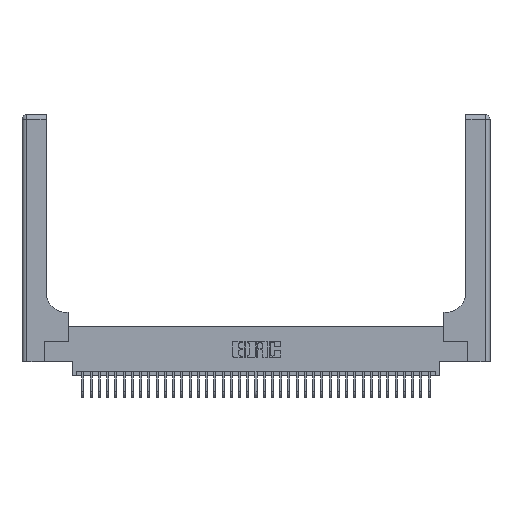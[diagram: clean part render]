
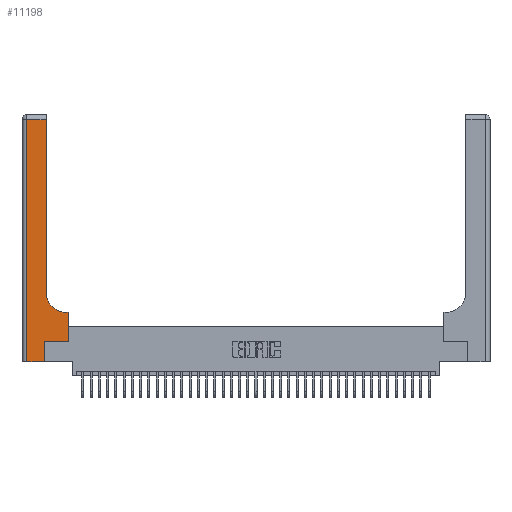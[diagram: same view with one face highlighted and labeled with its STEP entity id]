
A CAD part, top view. The second image highlights one B-rep face of the part: STEP entity #11198.
In plain terms, the highlighted planar face has unit normal (0, 0, 1).
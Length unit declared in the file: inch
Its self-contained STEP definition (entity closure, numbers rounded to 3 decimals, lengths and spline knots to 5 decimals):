
#14 = ORIENTED_EDGE ( 'NONE', *, *, #10716, .T. ) ;
#34 = VERTEX_POINT ( 'NONE', #37044 ) ;
#364 = EDGE_CURVE ( 'NONE', #31958, #33200, #26674, .T. ) ;
#442 = ORIENTED_EDGE ( 'NONE', *, *, #27554, .T. ) ;
#718 = VERTEX_POINT ( 'NONE', #11333 ) ;
#1422 = DIRECTION ( 'NONE',  ( -1., 0., 0. ) ) ;
#2027 = CARTESIAN_POINT ( 'NONE',  ( 0.5585, 0.6, 0.37 ) ) ;
#3683 = CARTESIAN_POINT ( 'NONE',  ( 0.5585, 0.25, 0.37 ) ) ;
#3736 = VERTEX_POINT ( 'NONE', #9401 ) ;
#4143 = CARTESIAN_POINT ( 'NONE',  ( 0.269, 0., 0.37 ) ) ;
#4271 = EDGE_CURVE ( 'NONE', #8091, #22768, #10926, .T. ) ;
#4682 = VERTEX_POINT ( 'NONE', #13950 ) ;
#6877 = CARTESIAN_POINT ( 'NONE',  ( 0.2915, 2.94, 0.37 ) ) ;
#7111 = DIRECTION ( 'NONE',  ( 0., 1., 0. ) ) ;
#7284 = EDGE_CURVE ( 'NONE', #4682, #8091, #32147, .T. ) ;
#7836 = VECTOR ( 'NONE', #7851, 39.37008 ) ;
#7851 = DIRECTION ( 'NONE',  ( -1., 0., 0. ) ) ;
#8091 = VERTEX_POINT ( 'NONE', #27769 ) ;
#8208 = CARTESIAN_POINT ( 'NONE',  ( 0.06, 3., 0.37 ) ) ;
#8946 = VECTOR ( 'NONE', #35458, 39.37008 ) ;
#8972 = EDGE_CURVE ( 'NONE', #34, #31958, #35555, .T. ) ;
#9401 = CARTESIAN_POINT ( 'NONE',  ( 0.2915, 0.85, 0.37 ) ) ;
#9494 = CARTESIAN_POINT ( 'NONE',  ( 0., 3., 0.37 ) ) ;
#9669 = DIRECTION ( 'NONE',  ( 1., 0., 0. ) ) ;
#9831 = CARTESIAN_POINT ( 'NONE',  ( 0.06, 0., 0.37 ) ) ;
#9869 = EDGE_CURVE ( 'NONE', #3736, #34813, #35478, .T. ) ;
#10716 = EDGE_CURVE ( 'NONE', #718, #3736, #24667, .T. ) ;
#10926 = LINE ( 'NONE', #3683, #24614 ) ;
#11183 = VECTOR ( 'NONE', #9669, 39.37008 ) ;
#11198 = ADVANCED_FACE ( 'NONE', ( #19751 ), #24074, .F. ) ;
#11333 = CARTESIAN_POINT ( 'NONE',  ( 0.5415, 0.6, 0.37 ) ) ;
#12494 = VECTOR ( 'NONE', #37082, 39.37008 ) ;
#12737 = VECTOR ( 'NONE', #1422, 39.37008 ) ;
#13571 = VECTOR ( 'NONE', #7111, 39.37008 ) ;
#13950 = CARTESIAN_POINT ( 'NONE',  ( 0.269, 0.25, 0.37 ) ) ;
#15389 = DIRECTION ( 'NONE',  ( -1., 0., 0. ) ) ;
#16310 = DIRECTION ( 'NONE',  ( 0., 0., -1. ) ) ;
#16577 = CARTESIAN_POINT ( 'NONE',  ( 0.2915, 3., 0.37 ) ) ;
#18393 = ORIENTED_EDGE ( 'NONE', *, *, #9869, .T. ) ;
#18813 = EDGE_CURVE ( 'NONE', #33200, #4682, #36606, .T. ) ;
#19751 = FACE_OUTER_BOUND ( 'NONE', #28714, .T. ) ;
#20494 = LINE ( 'NONE', #24713, #12737 ) ;
#21259 = DIRECTION ( 'NONE',  ( 0., 1., 0. ) ) ;
#22236 = AXIS2_PLACEMENT_3D ( 'NONE', #33645, #16310, #36498 ) ;
#22768 = VERTEX_POINT ( 'NONE', #2027 ) ;
#23400 = LINE ( 'NONE', #36853, #7836 ) ;
#23905 = EDGE_CURVE ( 'NONE', #34813, #34, #20494, .T. ) ;
#24074 = PLANE ( 'NONE',  #27341 ) ;
#24614 = VECTOR ( 'NONE', #21259, 39.37008 ) ;
#24667 = CIRCLE ( 'NONE', #22236, 0.25 ) ;
#24713 = CARTESIAN_POINT ( 'NONE',  ( 0., 2.94, 0.37 ) ) ;
#26674 = LINE ( 'NONE', #35755, #11183 ) ;
#26991 = VECTOR ( 'NONE', #33904, 39.37008 ) ;
#27341 = AXIS2_PLACEMENT_3D ( 'NONE', #9494, #32747, #15389 ) ;
#27554 = EDGE_CURVE ( 'NONE', #22768, #718, #23400, .T. ) ;
#27769 = CARTESIAN_POINT ( 'NONE',  ( 0.5585, 0.25, 0.37 ) ) ;
#28097 = ORIENTED_EDGE ( 'NONE', *, *, #18813, .T. ) ;
#28215 = ORIENTED_EDGE ( 'NONE', *, *, #4271, .T. ) ;
#28714 = EDGE_LOOP ( 'NONE', ( #18393, #33807, #33388, #35778, #28097, #28744, #28215, #442, #14 ) ) ;
#28744 = ORIENTED_EDGE ( 'NONE', *, *, #7284, .T. ) ;
#31313 = CARTESIAN_POINT ( 'NONE',  ( 0.269, 0., 0.37 ) ) ;
#31958 = VERTEX_POINT ( 'NONE', #9831 ) ;
#32147 = LINE ( 'NONE', #32619, #8946 ) ;
#32619 = CARTESIAN_POINT ( 'NONE',  ( 0.269, 0.25, 0.37 ) ) ;
#32747 = DIRECTION ( 'NONE',  ( 0., 0., -1. ) ) ;
#33200 = VERTEX_POINT ( 'NONE', #31313 ) ;
#33388 = ORIENTED_EDGE ( 'NONE', *, *, #8972, .T. ) ;
#33645 = CARTESIAN_POINT ( 'NONE',  ( 0.5415, 0.85, 0.37 ) ) ;
#33807 = ORIENTED_EDGE ( 'NONE', *, *, #23905, .T. ) ;
#33904 = DIRECTION ( 'NONE',  ( 0., 1., 0. ) ) ;
#34813 = VERTEX_POINT ( 'NONE', #6877 ) ;
#35458 = DIRECTION ( 'NONE',  ( 1., 0., 0. ) ) ;
#35478 = LINE ( 'NONE', #16577, #26991 ) ;
#35555 = LINE ( 'NONE', #8208, #12494 ) ;
#35755 = CARTESIAN_POINT ( 'NONE',  ( 0., 0., 0.37 ) ) ;
#35778 = ORIENTED_EDGE ( 'NONE', *, *, #364, .T. ) ;
#36498 = DIRECTION ( 'NONE',  ( 1., 0., 0. ) ) ;
#36606 = LINE ( 'NONE', #4143, #13571 ) ;
#36853 = CARTESIAN_POINT ( 'NONE',  ( 0.2915, 0.6, 0.37 ) ) ;
#37044 = CARTESIAN_POINT ( 'NONE',  ( 0.06, 2.94, 0.37 ) ) ;
#37082 = DIRECTION ( 'NONE',  ( 0., -1., 0. ) ) ;
